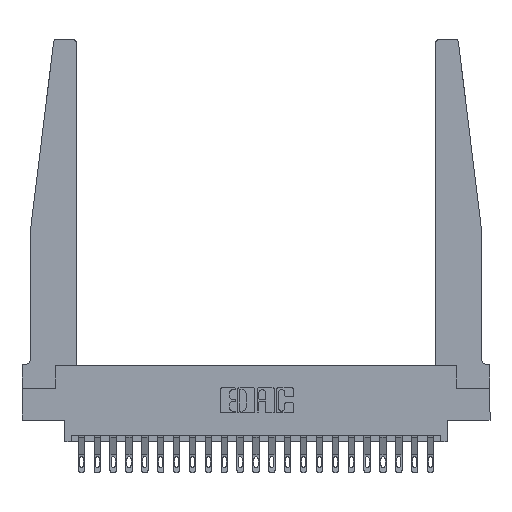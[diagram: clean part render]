
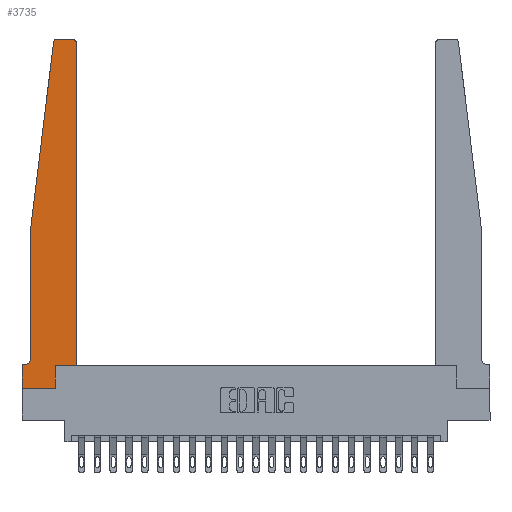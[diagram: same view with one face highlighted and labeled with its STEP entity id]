
A CAD part, top view. The second image highlights one B-rep face of the part: STEP entity #3735.
In plain terms, the highlighted planar face has unit normal (0, 0, 1).
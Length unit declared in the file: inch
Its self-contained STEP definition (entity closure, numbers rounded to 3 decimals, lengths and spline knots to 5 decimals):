
#266 = EDGE_CURVE ( 'NONE', #17232, #20583, #15778, .T. ) ;
#857 = ORIENTED_EDGE ( 'NONE', *, *, #266, .T. ) ;
#961 = DIRECTION ( 'NONE',  ( 0., 1., 0. ) ) ;
#1695 = VERTEX_POINT ( 'NONE', #17426 ) ;
#1815 = LINE ( 'NONE', #18729, #2361 ) ;
#2174 = DIRECTION ( 'NONE',  ( 0., 0., 1. ) ) ;
#2190 = VERTEX_POINT ( 'NONE', #9950 ) ;
#2361 = VECTOR ( 'NONE', #8185, 39.37008 ) ;
#2445 = ORIENTED_EDGE ( 'NONE', *, *, #18011, .T. ) ;
#2457 = AXIS2_PLACEMENT_3D ( 'NONE', #9141, #2174, #14521 ) ;
#2532 = CARTESIAN_POINT ( 'NONE',  ( 0., 0., 0.37 ) ) ;
#2788 = CARTESIAN_POINT ( 'NONE',  ( 0.27653, 2.72, 0.37 ) ) ;
#2905 = VECTOR ( 'NONE', #5724, 39.37008 ) ;
#3452 = LINE ( 'NONE', #12759, #2905 ) ;
#3456 = VERTEX_POINT ( 'NONE', #6835 ) ;
#3459 = ORIENTED_EDGE ( 'NONE', *, *, #11573, .T. ) ;
#3735 = ADVANCED_FACE ( 'NONE', ( #17275 ), #9205, .T. ) ;
#4006 = EDGE_CURVE ( 'NONE', #20663, #4087, #1815, .T. ) ;
#4087 = VERTEX_POINT ( 'NONE', #22367 ) ;
#4405 = LINE ( 'NONE', #9499, #22565 ) ;
#4546 = DIRECTION ( 'NONE',  ( 1., 0., 0. ) ) ;
#4829 = DIRECTION ( 'NONE',  ( 0., 0., -1. ) ) ;
#5218 = CARTESIAN_POINT ( 'NONE',  ( 0.015, 0.1875, 0.37 ) ) ;
#5401 = ORIENTED_EDGE ( 'NONE', *, *, #19940, .T. ) ;
#5724 = DIRECTION ( 'NONE',  ( 1., 0., 0. ) ) ;
#6835 = CARTESIAN_POINT ( 'NONE',  ( 0.425, 0.18, 0.37 ) ) ;
#7183 = AXIS2_PLACEMENT_3D ( 'NONE', #2788, #15119, #4546 ) ;
#7200 = VECTOR ( 'NONE', #20754, 39.37008 ) ;
#7294 = VERTEX_POINT ( 'NONE', #2532 ) ;
#7403 = EDGE_CURVE ( 'NONE', #3456, #21302, #22747, .T. ) ;
#8185 = DIRECTION ( 'NONE',  ( -1., 0., 0. ) ) ;
#8221 = CARTESIAN_POINT ( 'NONE',  ( 0., 0.1875, 0.37 ) ) ;
#8436 = DIRECTION ( 'NONE',  ( 0., 0., 1. ) ) ;
#8656 = CIRCLE ( 'NONE', #11426, 0.05 ) ;
#8799 = EDGE_LOOP ( 'NONE', ( #16191, #10012, #3459, #10461, #8927, #857, #20749, #10938, #5401, #2445, #20355, #16816 ) ) ;
#8927 = ORIENTED_EDGE ( 'NONE', *, *, #20080, .T. ) ;
#8973 = DIRECTION ( 'NONE',  ( 0., -1., 0. ) ) ;
#9089 = LINE ( 'NONE', #10725, #13220 ) ;
#9141 = CARTESIAN_POINT ( 'NONE',  ( 0., 0.1875, 0.37 ) ) ;
#9205 = PLANE ( 'NONE',  #2457 ) ;
#9499 = CARTESIAN_POINT ( 'NONE',  ( 0., 0., 0.37 ) ) ;
#9780 = CARTESIAN_POINT ( 'NONE',  ( 0.2605, 0.18, 0.37 ) ) ;
#9823 = VERTEX_POINT ( 'NONE', #18546 ) ;
#9950 = CARTESIAN_POINT ( 'NONE',  ( 0.24675, 2.72367, 0.37 ) ) ;
#10012 = ORIENTED_EDGE ( 'NONE', *, *, #22392, .T. ) ;
#10073 = EDGE_CURVE ( 'NONE', #20583, #7294, #21816, .T. ) ;
#10086 = DIRECTION ( 'NONE',  ( -1., 0., 0. ) ) ;
#10461 = ORIENTED_EDGE ( 'NONE', *, *, #13501, .T. ) ;
#10725 = CARTESIAN_POINT ( 'NONE',  ( 0.065, 1.25, 0.37 ) ) ;
#10862 = LINE ( 'NONE', #9780, #14991 ) ;
#10938 = ORIENTED_EDGE ( 'NONE', *, *, #22284, .T. ) ;
#11280 = CARTESIAN_POINT ( 'NONE',  ( 0.2605, 0.18, 0.37 ) ) ;
#11426 = AXIS2_PLACEMENT_3D ( 'NONE', #15390, #4829, #17155 ) ;
#11573 = EDGE_CURVE ( 'NONE', #2190, #9823, #21237, .T. ) ;
#12759 = CARTESIAN_POINT ( 'NONE',  ( 0.425, 0.18, 0.37 ) ) ;
#12908 = VECTOR ( 'NONE', #15186, 39.37008 ) ;
#13062 = DIRECTION ( 'NONE',  ( 1., 0., 0. ) ) ;
#13220 = VECTOR ( 'NONE', #8973, 39.37008 ) ;
#13501 = EDGE_CURVE ( 'NONE', #9823, #19443, #9089, .T. ) ;
#13595 = CARTESIAN_POINT ( 'NONE',  ( 0.065, 0.2375, 0.37 ) ) ;
#13680 = CARTESIAN_POINT ( 'NONE',  ( 0.425, 2.72, 0.37 ) ) ;
#13703 = CIRCLE ( 'NONE', #20336, 0.03 ) ;
#13782 = CARTESIAN_POINT ( 'NONE',  ( 0.395, 2.75, 0.37 ) ) ;
#14521 = DIRECTION ( 'NONE',  ( 1., 0., 0. ) ) ;
#14902 = CARTESIAN_POINT ( 'NONE',  ( 0.065, 0.1875, 0.37 ) ) ;
#14991 = VECTOR ( 'NONE', #961, 39.37008 ) ;
#15119 = DIRECTION ( 'NONE',  ( 0., 0., 1. ) ) ;
#15186 = DIRECTION ( 'NONE',  ( 0., 1., 0. ) ) ;
#15390 = CARTESIAN_POINT ( 'NONE',  ( 0.015, 0.2375, 0.37 ) ) ;
#15778 = LINE ( 'NONE', #14902, #19889 ) ;
#16068 = VECTOR ( 'NONE', #21870, 39.37008 ) ;
#16191 = ORIENTED_EDGE ( 'NONE', *, *, #4006, .T. ) ;
#16816 = ORIENTED_EDGE ( 'NONE', *, *, #17705, .T. ) ;
#17155 = DIRECTION ( 'NONE',  ( -1., 0., 0. ) ) ;
#17232 = VERTEX_POINT ( 'NONE', #5218 ) ;
#17275 = FACE_OUTER_BOUND ( 'NONE', #8799, .T. ) ;
#17426 = CARTESIAN_POINT ( 'NONE',  ( 0.2605, 0., 0.37 ) ) ;
#17705 = EDGE_CURVE ( 'NONE', #21302, #20663, #13703, .T. ) ;
#18011 = EDGE_CURVE ( 'NONE', #21069, #3456, #3452, .T. ) ;
#18546 = CARTESIAN_POINT ( 'NONE',  ( 0.065, 1.25, 0.37 ) ) ;
#18643 = CARTESIAN_POINT ( 'NONE',  ( 0.425, 0.18, 0.37 ) ) ;
#18729 = CARTESIAN_POINT ( 'NONE',  ( 0.25, 2.75, 0.37 ) ) ;
#18986 = CARTESIAN_POINT ( 'NONE',  ( 0.395, 2.72, 0.37 ) ) ;
#19443 = VERTEX_POINT ( 'NONE', #13595 ) ;
#19889 = VECTOR ( 'NONE', #10086, 39.37008 ) ;
#19940 = EDGE_CURVE ( 'NONE', #1695, #21069, #10862, .T. ) ;
#20080 = EDGE_CURVE ( 'NONE', #19443, #17232, #8656, .T. ) ;
#20124 = CARTESIAN_POINT ( 'NONE',  ( 0., 0., 0.37 ) ) ;
#20336 = AXIS2_PLACEMENT_3D ( 'NONE', #18986, #8436, #20740 ) ;
#20355 = ORIENTED_EDGE ( 'NONE', *, *, #7403, .T. ) ;
#20583 = VERTEX_POINT ( 'NONE', #8221 ) ;
#20663 = VERTEX_POINT ( 'NONE', #13782 ) ;
#20679 = CARTESIAN_POINT ( 'NONE',  ( 0.065, 1.25, 0.37 ) ) ;
#20740 = DIRECTION ( 'NONE',  ( 1., 0., 0. ) ) ;
#20749 = ORIENTED_EDGE ( 'NONE', *, *, #10073, .T. ) ;
#20754 = DIRECTION ( 'NONE',  ( -0.122, -0.992, 0. ) ) ;
#21069 = VERTEX_POINT ( 'NONE', #11280 ) ;
#21237 = LINE ( 'NONE', #20679, #7200 ) ;
#21302 = VERTEX_POINT ( 'NONE', #13680 ) ;
#21490 = CIRCLE ( 'NONE', #7183, 0.03 ) ;
#21816 = LINE ( 'NONE', #20124, #16068 ) ;
#21870 = DIRECTION ( 'NONE',  ( 0., -1., 0. ) ) ;
#22284 = EDGE_CURVE ( 'NONE', #7294, #1695, #4405, .T. ) ;
#22367 = CARTESIAN_POINT ( 'NONE',  ( 0.27653, 2.75, 0.37 ) ) ;
#22392 = EDGE_CURVE ( 'NONE', #4087, #2190, #21490, .T. ) ;
#22565 = VECTOR ( 'NONE', #13062, 39.37008 ) ;
#22747 = LINE ( 'NONE', #18643, #12908 ) ;
